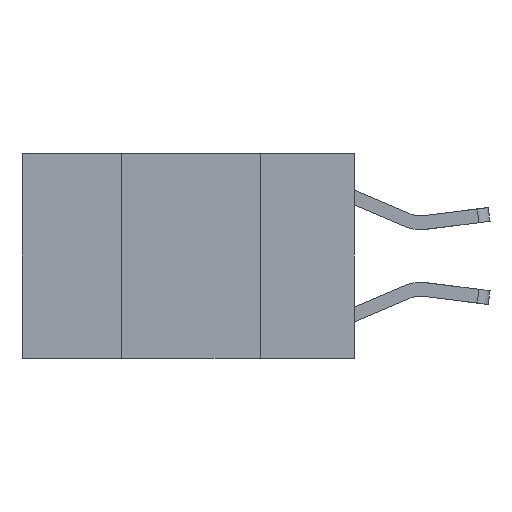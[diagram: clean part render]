
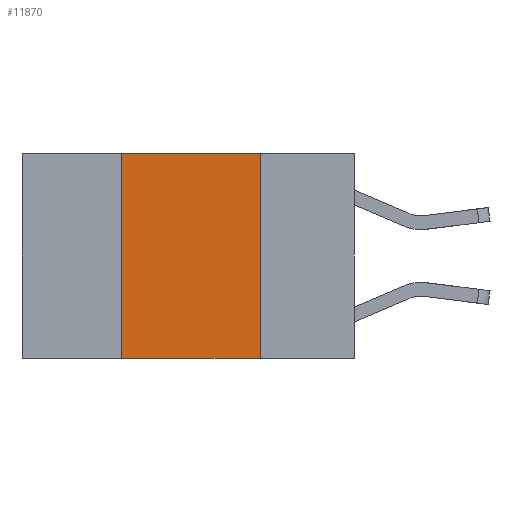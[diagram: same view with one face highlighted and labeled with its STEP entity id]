
A CAD part, left-side view. The second image highlights one B-rep face of the part: STEP entity #11870.
In plain terms, the highlighted planar face has unit normal (-1, 0, 0).
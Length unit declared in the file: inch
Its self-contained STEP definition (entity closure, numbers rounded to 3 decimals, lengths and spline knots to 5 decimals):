
#158 = ORIENTED_EDGE ( 'NONE', *, *, #9934, .F. ) ;
#536 = CARTESIAN_POINT ( 'NONE',  ( 0., 0.42, -0.37 ) ) ;
#938 = LINE ( 'NONE', #4922, #4738 ) ;
#942 = DIRECTION ( 'NONE',  ( 0., -1., 0. ) ) ;
#1478 = DIRECTION ( 'NONE',  ( 0., 0., -1. ) ) ;
#1731 = VECTOR ( 'NONE', #6132, 39.37008 ) ;
#2517 = FACE_OUTER_BOUND ( 'NONE', #6843, .T. ) ;
#2874 = VERTEX_POINT ( 'NONE', #6210 ) ;
#3220 = CARTESIAN_POINT ( 'NONE',  ( 0., 0.6, -0.37 ) ) ;
#3264 = DIRECTION ( 'NONE',  ( 1., 0., 0. ) ) ;
#3985 = DIRECTION ( 'NONE',  ( 0., 0., 1. ) ) ;
#4527 = VERTEX_POINT ( 'NONE', #4999 ) ;
#4738 = VECTOR ( 'NONE', #3985, 39.37008 ) ;
#4840 = CARTESIAN_POINT ( 'NONE',  ( 0., 0.17, 0. ) ) ;
#4922 = CARTESIAN_POINT ( 'NONE',  ( 0., 0.42, 0. ) ) ;
#4980 = CARTESIAN_POINT ( 'NONE',  ( 0., 0.17, 0. ) ) ;
#4999 = CARTESIAN_POINT ( 'NONE',  ( 0., 0.17, -0.37 ) ) ;
#5412 = VERTEX_POINT ( 'NONE', #536 ) ;
#5878 = DIRECTION ( 'NONE',  ( 0., 0., -1. ) ) ;
#6132 = DIRECTION ( 'NONE',  ( 0., -1., 0. ) ) ;
#6210 = CARTESIAN_POINT ( 'NONE',  ( 0., 0.42, 0. ) ) ;
#6361 = VECTOR ( 'NONE', #5878, 39.37008 ) ;
#6448 = ORIENTED_EDGE ( 'NONE', *, *, #8088, .T. ) ;
#6563 = EDGE_CURVE ( 'NONE', #5412, #2874, #938, .T. ) ;
#6775 = LINE ( 'NONE', #12326, #10764 ) ;
#6843 = EDGE_LOOP ( 'NONE', ( #8597, #158, #8688, #6448 ) ) ;
#7035 = EDGE_CURVE ( 'NONE', #11707, #4527, #8817, .T. ) ;
#8088 = EDGE_CURVE ( 'NONE', #5412, #4527, #11945, .T. ) ;
#8131 = CARTESIAN_POINT ( 'NONE',  ( 0., 0.6, 0. ) ) ;
#8258 = PLANE ( 'NONE',  #12331 ) ;
#8597 = ORIENTED_EDGE ( 'NONE', *, *, #7035, .F. ) ;
#8688 = ORIENTED_EDGE ( 'NONE', *, *, #6563, .F. ) ;
#8817 = LINE ( 'NONE', #4840, #6361 ) ;
#9934 = EDGE_CURVE ( 'NONE', #2874, #11707, #6775, .T. ) ;
#10764 = VECTOR ( 'NONE', #942, 39.37008 ) ;
#11707 = VERTEX_POINT ( 'NONE', #4980 ) ;
#11870 = ADVANCED_FACE ( 'NONE', ( #2517 ), #8258, .F. ) ;
#11945 = LINE ( 'NONE', #3220, #1731 ) ;
#12326 = CARTESIAN_POINT ( 'NONE',  ( 0., 0.6, 0. ) ) ;
#12331 = AXIS2_PLACEMENT_3D ( 'NONE', #8131, #3264, #1478 ) ;
